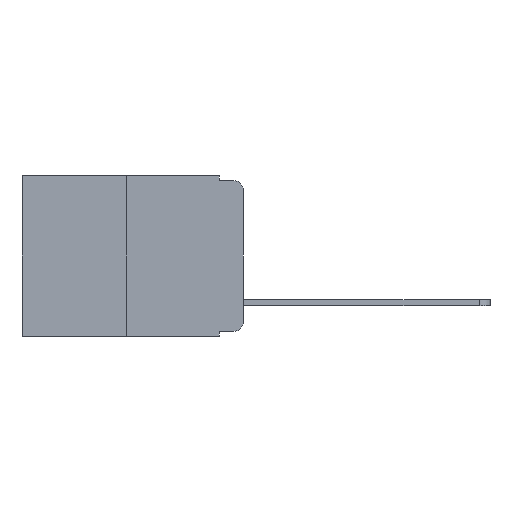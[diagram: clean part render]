
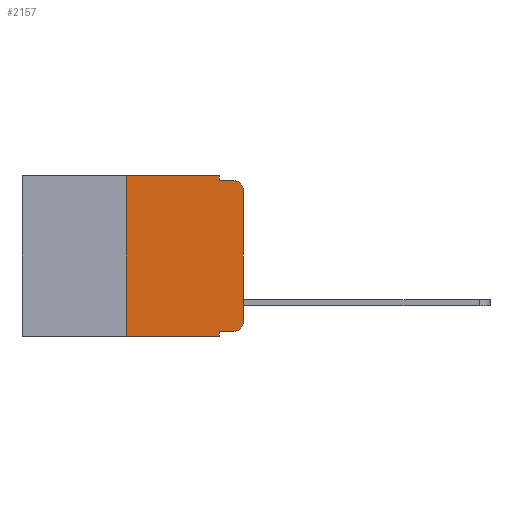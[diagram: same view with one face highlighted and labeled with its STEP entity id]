
A CAD part, left-side view. The second image highlights one B-rep face of the part: STEP entity #2157.
In plain terms, the highlighted planar face has unit normal (-1, 0, 0).
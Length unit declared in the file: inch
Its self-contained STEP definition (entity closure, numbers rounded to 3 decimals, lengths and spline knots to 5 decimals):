
#68 = CIRCLE ( 'NONE', #1555, 0.02 ) ;
#206 = AXIS2_PLACEMENT_3D ( 'NONE', #4763, #7278, #1416 ) ;
#535 = CARTESIAN_POINT ( 'NONE',  ( 0., 0., 0. ) ) ;
#660 = LINE ( 'NONE', #4285, #8173 ) ;
#1014 = LINE ( 'NONE', #5235, #6633 ) ;
#1127 = VERTEX_POINT ( 'NONE', #4643 ) ;
#1199 = EDGE_CURVE ( 'NONE', #8443, #4752, #5525, .T. ) ;
#1416 = DIRECTION ( 'NONE',  ( 0., 0., -1. ) ) ;
#1555 = AXIS2_PLACEMENT_3D ( 'NONE', #2899, #2940, #2950 ) ;
#1560 = VECTOR ( 'NONE', #6325, 39.37008 ) ;
#1591 = VERTEX_POINT ( 'NONE', #3114 ) ;
#1754 = ORIENTED_EDGE ( 'NONE', *, *, #3966, .F. ) ;
#1839 = LINE ( 'NONE', #7556, #9217 ) ;
#2091 = EDGE_CURVE ( 'NONE', #8563, #2850, #660, .T. ) ;
#2157 = ADVANCED_FACE ( 'NONE', ( #7959 ), #4828, .F. ) ;
#2295 = AXIS2_PLACEMENT_3D ( 'NONE', #7422, #7416, #7414 ) ;
#2359 = DIRECTION ( 'NONE',  ( 0., -1., 0. ) ) ;
#2397 = EDGE_CURVE ( 'NONE', #8563, #5716, #7547, .T. ) ;
#2484 = CARTESIAN_POINT ( 'NONE',  ( 0., 0.25, 0. ) ) ;
#2587 = CIRCLE ( 'NONE', #2295, 0.02 ) ;
#2809 = CARTESIAN_POINT ( 'NONE',  ( 0., 0.02, -0.333 ) ) ;
#2850 = VERTEX_POINT ( 'NONE', #6679 ) ;
#2899 = CARTESIAN_POINT ( 'NONE',  ( 0., 0.02, -0.03 ) ) ;
#2906 = ORIENTED_EDGE ( 'NONE', *, *, #8367, .T. ) ;
#2916 = ORIENTED_EDGE ( 'NONE', *, *, #1199, .T. ) ;
#2940 = DIRECTION ( 'NONE',  ( -1., 0., 0. ) ) ;
#2950 = DIRECTION ( 'NONE',  ( 0., 0., -1. ) ) ;
#3098 = CARTESIAN_POINT ( 'NONE',  ( 0., 0.051, -0.01 ) ) ;
#3114 = CARTESIAN_POINT ( 'NONE',  ( 0., 0.051, -0.333 ) ) ;
#3196 = DIRECTION ( 'NONE',  ( 0., -1., 0. ) ) ;
#3204 = LINE ( 'NONE', #5013, #8469 ) ;
#3658 = EDGE_CURVE ( 'NONE', #1591, #2850, #1839, .T. ) ;
#3869 = EDGE_LOOP ( 'NONE', ( #2916, #2906, #1754, #8135, #7439, #5242, #6939, #8861, #8968, #7760 ) ) ;
#3966 = EDGE_CURVE ( 'NONE', #1127, #7987, #5622, .T. ) ;
#4285 = CARTESIAN_POINT ( 'NONE',  ( 0., 0.473, -0.343 ) ) ;
#4332 = CARTESIAN_POINT ( 'NONE',  ( 0., 0., -0.313 ) ) ;
#4362 = DIRECTION ( 'NONE',  ( 0., -1., 0. ) ) ;
#4643 = CARTESIAN_POINT ( 'NONE',  ( 0., 0.051, -0.01 ) ) ;
#4752 = VERTEX_POINT ( 'NONE', #7109 ) ;
#4763 = CARTESIAN_POINT ( 'NONE',  ( 0., 0.473, 0. ) ) ;
#4828 = PLANE ( 'NONE',  #206 ) ;
#5013 = CARTESIAN_POINT ( 'NONE',  ( 0., 0.051, 0. ) ) ;
#5235 = CARTESIAN_POINT ( 'NONE',  ( 0., 0.051, -0.333 ) ) ;
#5242 = ORIENTED_EDGE ( 'NONE', *, *, #2397, .F. ) ;
#5357 = EDGE_CURVE ( 'NONE', #6824, #1127, #3204, .T. ) ;
#5413 = VECTOR ( 'NONE', #3196, 39.37008 ) ;
#5525 = LINE ( 'NONE', #535, #5753 ) ;
#5605 = VERTEX_POINT ( 'NONE', #2809 ) ;
#5622 = LINE ( 'NONE', #3098, #5413 ) ;
#5645 = VECTOR ( 'NONE', #6815, 39.37008 ) ;
#5716 = VERTEX_POINT ( 'NONE', #8608 ) ;
#5753 = VECTOR ( 'NONE', #9154, 39.37008 ) ;
#6325 = DIRECTION ( 'NONE',  ( 0., -1., 0. ) ) ;
#6571 = EDGE_CURVE ( 'NONE', #1591, #5605, #1014, .T. ) ;
#6633 = VECTOR ( 'NONE', #4362, 39.37008 ) ;
#6679 = CARTESIAN_POINT ( 'NONE',  ( 0., 0.051, -0.343 ) ) ;
#6815 = DIRECTION ( 'NONE',  ( 0., 0., 1. ) ) ;
#6824 = VERTEX_POINT ( 'NONE', #8306 ) ;
#6939 = ORIENTED_EDGE ( 'NONE', *, *, #2091, .T. ) ;
#7069 = EDGE_CURVE ( 'NONE', #5716, #6824, #8973, .T. ) ;
#7109 = CARTESIAN_POINT ( 'NONE',  ( 0., 0., -0.03 ) ) ;
#7193 = EDGE_CURVE ( 'NONE', #5605, #8443, #2587, .T. ) ;
#7278 = DIRECTION ( 'NONE',  ( 1., 0., 0. ) ) ;
#7414 = DIRECTION ( 'NONE',  ( 0., 0., -1. ) ) ;
#7416 = DIRECTION ( 'NONE',  ( -1., 0., 0. ) ) ;
#7422 = CARTESIAN_POINT ( 'NONE',  ( 0., 0.02, -0.313 ) ) ;
#7439 = ORIENTED_EDGE ( 'NONE', *, *, #7069, .F. ) ;
#7547 = LINE ( 'NONE', #2484, #5645 ) ;
#7556 = CARTESIAN_POINT ( 'NONE',  ( 0., 0.051, 0. ) ) ;
#7588 = DIRECTION ( 'NONE',  ( 0., 0., -1. ) ) ;
#7760 = ORIENTED_EDGE ( 'NONE', *, *, #7193, .T. ) ;
#7846 = CARTESIAN_POINT ( 'NONE',  ( 0., 0.473, 0. ) ) ;
#7895 = CARTESIAN_POINT ( 'NONE',  ( 0., 0.25, -0.343 ) ) ;
#7959 = FACE_OUTER_BOUND ( 'NONE', #3869, .T. ) ;
#7987 = VERTEX_POINT ( 'NONE', #9101 ) ;
#8135 = ORIENTED_EDGE ( 'NONE', *, *, #5357, .F. ) ;
#8173 = VECTOR ( 'NONE', #2359, 39.37008 ) ;
#8306 = CARTESIAN_POINT ( 'NONE',  ( 0., 0.051, 0. ) ) ;
#8367 = EDGE_CURVE ( 'NONE', #4752, #7987, #68, .T. ) ;
#8443 = VERTEX_POINT ( 'NONE', #4332 ) ;
#8469 = VECTOR ( 'NONE', #8626, 39.37008 ) ;
#8563 = VERTEX_POINT ( 'NONE', #7895 ) ;
#8608 = CARTESIAN_POINT ( 'NONE',  ( 0., 0.25, 0. ) ) ;
#8626 = DIRECTION ( 'NONE',  ( 0., 0., -1. ) ) ;
#8861 = ORIENTED_EDGE ( 'NONE', *, *, #3658, .F. ) ;
#8968 = ORIENTED_EDGE ( 'NONE', *, *, #6571, .T. ) ;
#8973 = LINE ( 'NONE', #7846, #1560 ) ;
#9101 = CARTESIAN_POINT ( 'NONE',  ( 0., 0.02, -0.01 ) ) ;
#9154 = DIRECTION ( 'NONE',  ( 0., 0., 1. ) ) ;
#9217 = VECTOR ( 'NONE', #7588, 39.37008 ) ;
